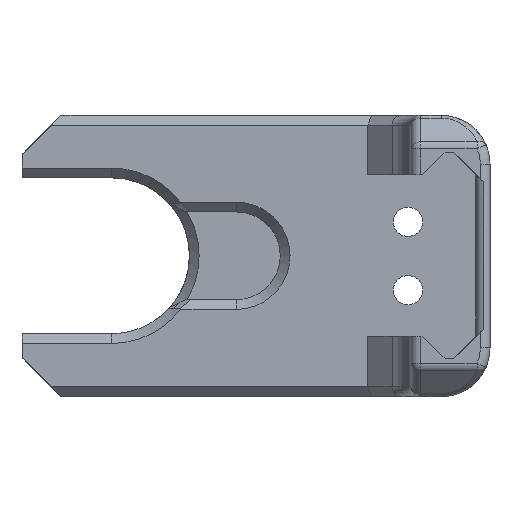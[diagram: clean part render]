
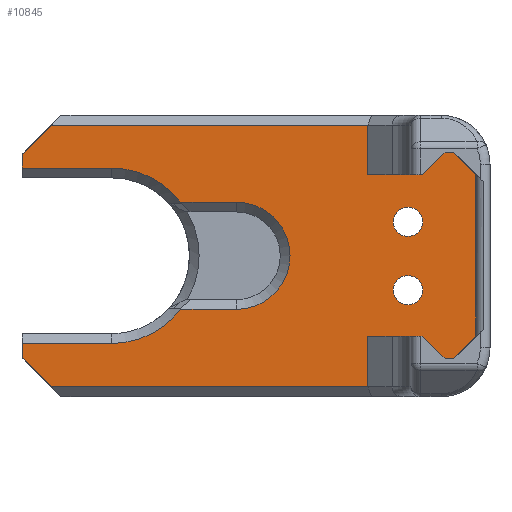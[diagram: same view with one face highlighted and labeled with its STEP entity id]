
A CAD part, left-side view. The second image highlights one B-rep face of the part: STEP entity #10845.
In plain terms, the highlighted planar face has unit normal (-1, 0, 0).
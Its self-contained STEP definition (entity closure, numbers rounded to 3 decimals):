
#565=FACE_BOUND('',#2460,.T.);
#566=FACE_BOUND('',#2461,.T.);
#589=CIRCLE('',#11524,9.);
#590=CIRCLE('',#11525,5.5);
#591=CIRCLE('',#11526,9.);
#592=CIRCLE('',#11527,1.5);
#593=CIRCLE('',#11528,1.5);
#676=PLANE('',#11523);
#1738=FACE_OUTER_BOUND('',#2459,.T.);
#2459=EDGE_LOOP('',(#7876,#7877,#7878,#7879,#7880,#7881,#7882,#7883,#7884,
#7885,#7886,#7887,#7888,#7889,#7890,#7891,#7892,#7893,#7894,#7895,#7896,
#7897,#7898,#7899));
#2460=EDGE_LOOP('',(#7900));
#2461=EDGE_LOOP('',(#7901));
#3163=LINE('',#15581,#3847);
#3164=LINE('',#15583,#3848);
#3165=LINE('',#15585,#3849);
#3166=LINE('',#15587,#3850);
#3167=LINE('',#15589,#3851);
#3168=LINE('',#15591,#3852);
#3169=LINE('',#15593,#3853);
#3170=LINE('',#15595,#3854);
#3171=LINE('',#15599,#3855);
#3172=LINE('',#15603,#3856);
#3173=LINE('',#15607,#3857);
#3174=LINE('',#15609,#3858);
#3175=LINE('',#15611,#3859);
#3176=LINE('',#15613,#3860);
#3177=LINE('',#15615,#3861);
#3178=LINE('',#15617,#3862);
#3179=LINE('',#15619,#3863);
#3180=LINE('',#15621,#3864);
#3181=LINE('',#15623,#3865);
#3182=LINE('',#15625,#3866);
#3183=LINE('',#15626,#3867);
#3847=VECTOR('',#11915,10.);
#3848=VECTOR('',#11916,10.);
#3849=VECTOR('',#11917,10.);
#3850=VECTOR('',#11918,10.);
#3851=VECTOR('',#11919,10.);
#3852=VECTOR('',#11920,10.);
#3853=VECTOR('',#11921,10.);
#3854=VECTOR('',#11922,10.);
#3855=VECTOR('',#11925,10.);
#3856=VECTOR('',#11928,10.);
#3857=VECTOR('',#11931,10.);
#3858=VECTOR('',#11932,10.);
#3859=VECTOR('',#11933,10.);
#3860=VECTOR('',#11934,10.);
#3861=VECTOR('',#11935,10.);
#3862=VECTOR('',#11936,10.);
#3863=VECTOR('',#11937,10.);
#3864=VECTOR('',#11938,10.);
#3865=VECTOR('',#11939,10.);
#3866=VECTOR('',#11940,10.);
#3867=VECTOR('',#11941,10.);
#4986=VERTEX_POINT('',#15579);
#4987=VERTEX_POINT('',#15580);
#4988=VERTEX_POINT('',#15582);
#4989=VERTEX_POINT('',#15584);
#4990=VERTEX_POINT('',#15586);
#4991=VERTEX_POINT('',#15588);
#4992=VERTEX_POINT('',#15590);
#4993=VERTEX_POINT('',#15592);
#4994=VERTEX_POINT('',#15594);
#4995=VERTEX_POINT('',#15596);
#4996=VERTEX_POINT('',#15598);
#4997=VERTEX_POINT('',#15600);
#4998=VERTEX_POINT('',#15602);
#4999=VERTEX_POINT('',#15604);
#5000=VERTEX_POINT('',#15606);
#5001=VERTEX_POINT('',#15608);
#5002=VERTEX_POINT('',#15610);
#5003=VERTEX_POINT('',#15612);
#5004=VERTEX_POINT('',#15614);
#5005=VERTEX_POINT('',#15616);
#5006=VERTEX_POINT('',#15618);
#5007=VERTEX_POINT('',#15620);
#5008=VERTEX_POINT('',#15622);
#5009=VERTEX_POINT('',#15624);
#5010=VERTEX_POINT('',#15627);
#5011=VERTEX_POINT('',#15629);
#6140=EDGE_CURVE('',#4986,#4987,#3163,.T.);
#6141=EDGE_CURVE('',#4986,#4988,#3164,.T.);
#6142=EDGE_CURVE('',#4988,#4989,#3165,.T.);
#6143=EDGE_CURVE('',#4990,#4989,#3166,.T.);
#6144=EDGE_CURVE('',#4991,#4990,#3167,.T.);
#6145=EDGE_CURVE('',#4992,#4991,#3168,.T.);
#6146=EDGE_CURVE('',#4992,#4993,#3169,.T.);
#6147=EDGE_CURVE('',#4994,#4993,#3170,.T.);
#6148=EDGE_CURVE('',#4995,#4994,#589,.T.);
#6149=EDGE_CURVE('',#4996,#4995,#3171,.T.);
#6150=EDGE_CURVE('',#4997,#4996,#590,.T.);
#6151=EDGE_CURVE('',#4998,#4997,#3172,.T.);
#6152=EDGE_CURVE('',#4999,#4998,#591,.T.);
#6153=EDGE_CURVE('',#5000,#4999,#3173,.T.);
#6154=EDGE_CURVE('',#5000,#5001,#3174,.T.);
#6155=EDGE_CURVE('',#5002,#5001,#3175,.T.);
#6156=EDGE_CURVE('',#5003,#5002,#3176,.T.);
#6157=EDGE_CURVE('',#5004,#5003,#3177,.T.);
#6158=EDGE_CURVE('',#5004,#5005,#3178,.T.);
#6159=EDGE_CURVE('',#5006,#5005,#3179,.T.);
#6160=EDGE_CURVE('',#5007,#5006,#3180,.T.);
#6161=EDGE_CURVE('',#5008,#5007,#3181,.T.);
#6162=EDGE_CURVE('',#5009,#5008,#3182,.T.);
#6163=EDGE_CURVE('',#4987,#5009,#3183,.T.);
#6164=EDGE_CURVE('',#5010,#5010,#592,.T.);
#6165=EDGE_CURVE('',#5011,#5011,#593,.T.);
#7876=ORIENTED_EDGE('',*,*,#6140,.F.);
#7877=ORIENTED_EDGE('',*,*,#6141,.T.);
#7878=ORIENTED_EDGE('',*,*,#6142,.T.);
#7879=ORIENTED_EDGE('',*,*,#6143,.F.);
#7880=ORIENTED_EDGE('',*,*,#6144,.F.);
#7881=ORIENTED_EDGE('',*,*,#6145,.F.);
#7882=ORIENTED_EDGE('',*,*,#6146,.T.);
#7883=ORIENTED_EDGE('',*,*,#6147,.F.);
#7884=ORIENTED_EDGE('',*,*,#6148,.F.);
#7885=ORIENTED_EDGE('',*,*,#6149,.F.);
#7886=ORIENTED_EDGE('',*,*,#6150,.F.);
#7887=ORIENTED_EDGE('',*,*,#6151,.F.);
#7888=ORIENTED_EDGE('',*,*,#6152,.F.);
#7889=ORIENTED_EDGE('',*,*,#6153,.F.);
#7890=ORIENTED_EDGE('',*,*,#6154,.T.);
#7891=ORIENTED_EDGE('',*,*,#6155,.F.);
#7892=ORIENTED_EDGE('',*,*,#6156,.F.);
#7893=ORIENTED_EDGE('',*,*,#6157,.F.);
#7894=ORIENTED_EDGE('',*,*,#6158,.T.);
#7895=ORIENTED_EDGE('',*,*,#6159,.F.);
#7896=ORIENTED_EDGE('',*,*,#6160,.F.);
#7897=ORIENTED_EDGE('',*,*,#6161,.F.);
#7898=ORIENTED_EDGE('',*,*,#6162,.F.);
#7899=ORIENTED_EDGE('',*,*,#6163,.F.);
#7900=ORIENTED_EDGE('',*,*,#6164,.T.);
#7901=ORIENTED_EDGE('',*,*,#6165,.T.);
#10845=ADVANCED_FACE('',(#1738,#565,#566),#676,.F.);
#11523=AXIS2_PLACEMENT_3D('',#15578,#11913,#11914);
#11524=AXIS2_PLACEMENT_3D('',#15597,#11923,#11924);
#11525=AXIS2_PLACEMENT_3D('',#15601,#11926,#11927);
#11526=AXIS2_PLACEMENT_3D('',#15605,#11929,#11930);
#11527=AXIS2_PLACEMENT_3D('',#15628,#11942,#11943);
#11528=AXIS2_PLACEMENT_3D('',#15630,#11944,#11945);
#11913=DIRECTION('center_axis',(1.,0.,0.));
#11914=DIRECTION('ref_axis',(0.,1.,0.));
#11915=DIRECTION('',(0.,-1.,0.));
#11916=DIRECTION('',(0.,0.707,-0.707));
#11917=DIRECTION('',(0.,1.,0.));
#11918=DIRECTION('',(0.,0.,-1.));
#11919=DIRECTION('',(0.,-1.,0.));
#11920=DIRECTION('',(0.,-0.707,0.707));
#11921=DIRECTION('',(0.,0.,-1.));
#11922=DIRECTION('',(0.,1.,0.));
#11923=DIRECTION('center_axis',(-1.,0.,0.));
#11924=DIRECTION('ref_axis',(0.,-1.,0.));
#11925=DIRECTION('',(0.,1.,0.));
#11926=DIRECTION('center_axis',(-1.,0.,0.));
#11927=DIRECTION('ref_axis',(0.,-1.,0.));
#11928=DIRECTION('',(0.,-1.,0.));
#11929=DIRECTION('center_axis',(-1.,0.,0.));
#11930=DIRECTION('ref_axis',(0.,-1.,0.));
#11931=DIRECTION('',(0.,-1.,0.));
#11932=DIRECTION('',(0.,0.,-1.));
#11933=DIRECTION('',(0.,0.707,0.707));
#11934=DIRECTION('',(0.,1.,0.));
#11935=DIRECTION('',(0.,0.,-1.));
#11936=DIRECTION('',(0.,-1.,0.));
#11937=DIRECTION('',(0.,0.707,0.707));
#11938=DIRECTION('',(0.,1.,0.));
#11939=DIRECTION('',(0.,0.707,-0.707));
#11940=DIRECTION('',(0.,0.,-1.));
#11941=DIRECTION('',(0.,-0.707,-0.707));
#11942=DIRECTION('center_axis',(1.,0.,0.));
#11943=DIRECTION('ref_axis',(0.,1.,0.));
#11944=DIRECTION('center_axis',(1.,0.,0.));
#11945=DIRECTION('ref_axis',(0.,1.,0.));
#15578=CARTESIAN_POINT('Origin',(172.686,-3.016,-0.022));
#15579=CARTESIAN_POINT('',(172.686,-22.914,10.612));
#15580=CARTESIAN_POINT('',(172.686,-23.822,10.612));
#15581=CARTESIAN_POINT('',(172.686,-13.106,10.612));
#15582=CARTESIAN_POINT('',(172.686,-20.639,8.337));
#15583=CARTESIAN_POINT('',(172.686,-14.229,1.927));
#15584=CARTESIAN_POINT('',(172.686,-14.983,8.337));
#15585=CARTESIAN_POINT('',(172.686,-10.249,8.337));
#15586=CARTESIAN_POINT('',(172.686,-14.983,13.409));
#15587=CARTESIAN_POINT('',(172.686,-14.983,7.193));
#15588=CARTESIAN_POINT('',(172.686,17.5,13.409));
#15589=CARTESIAN_POINT('',(172.686,-2.258,13.409));
#15590=CARTESIAN_POINT('',(172.686,20.5,10.409));
#15591=CARTESIAN_POINT('',(172.686,16.229,14.68));
#15592=CARTESIAN_POINT('',(172.686,20.5,9.));
#15593=CARTESIAN_POINT('',(172.686,20.5,-7.238));
#15594=CARTESIAN_POINT('',(172.686,11.317,9.));
#15595=CARTESIAN_POINT('',(172.686,9.242,9.));
#15596=CARTESIAN_POINT('',(172.686,4.193,5.5));
#15597=CARTESIAN_POINT('Origin',(172.686,11.317,0.));
#15598=CARTESIAN_POINT('',(172.686,-1.506,5.5));
#15599=CARTESIAN_POINT('',(172.686,1.203,5.5));
#15600=CARTESIAN_POINT('',(172.686,-1.506,-5.5));
#15601=CARTESIAN_POINT('Origin',(172.686,-1.506,0.));
#15602=CARTESIAN_POINT('',(172.686,4.193,-5.5));
#15603=CARTESIAN_POINT('',(172.686,-2.261,-5.5));
#15604=CARTESIAN_POINT('',(172.686,11.317,-9.));
#15605=CARTESIAN_POINT('Origin',(172.686,11.317,0.));
#15606=CARTESIAN_POINT('',(172.686,20.5,-9.));
#15607=CARTESIAN_POINT('',(172.686,4.15,-9.));
#15608=CARTESIAN_POINT('',(172.686,20.5,-10.453));
#15609=CARTESIAN_POINT('',(172.686,20.5,-7.238));
#15610=CARTESIAN_POINT('',(172.686,17.5,-13.453));
#15611=CARTESIAN_POINT('',(172.686,16.229,-14.724));
#15612=CARTESIAN_POINT('',(172.686,-14.983,-13.453));
#15613=CARTESIAN_POINT('',(172.686,-15.273,-13.453));
#15614=CARTESIAN_POINT('',(172.686,-14.983,-8.263));
#15615=CARTESIAN_POINT('',(172.686,-14.983,-3.893));
#15616=CARTESIAN_POINT('',(172.686,-20.591,-8.263));
#15617=CARTESIAN_POINT('',(172.686,-11.984,-8.263));
#15618=CARTESIAN_POINT('',(172.686,-22.917,-10.589));
#15619=CARTESIAN_POINT('',(172.686,-15.37,-3.043));
#15620=CARTESIAN_POINT('',(172.686,-23.822,-10.589));
#15621=CARTESIAN_POINT('',(172.686,-13.419,-10.589));
#15622=CARTESIAN_POINT('',(172.686,-26.066,-8.346));
#15623=CARTESIAN_POINT('',(172.686,-22.384,-12.027));
#15624=CARTESIAN_POINT('',(172.686,-26.066,8.368));
#15625=CARTESIAN_POINT('',(172.686,-26.066,4.173));
#15626=CARTESIAN_POINT('',(172.686,-21.279,13.155));
#15627=CARTESIAN_POINT('',(172.686,-20.61,3.478));
#15628=CARTESIAN_POINT('Origin',(172.686,-19.11,3.478));
#15629=CARTESIAN_POINT('',(172.686,-20.61,-3.522));
#15630=CARTESIAN_POINT('Origin',(172.686,-19.11,-3.522));
